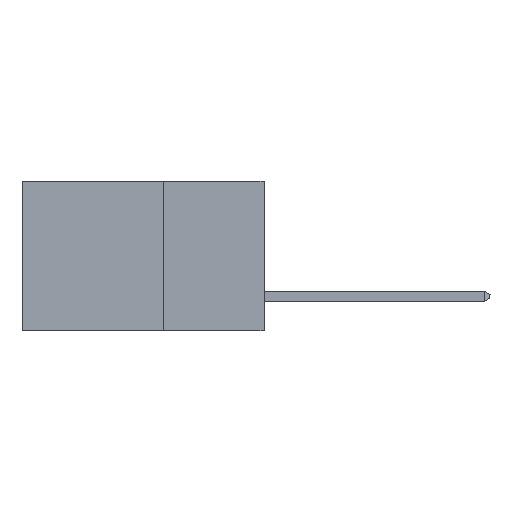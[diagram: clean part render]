
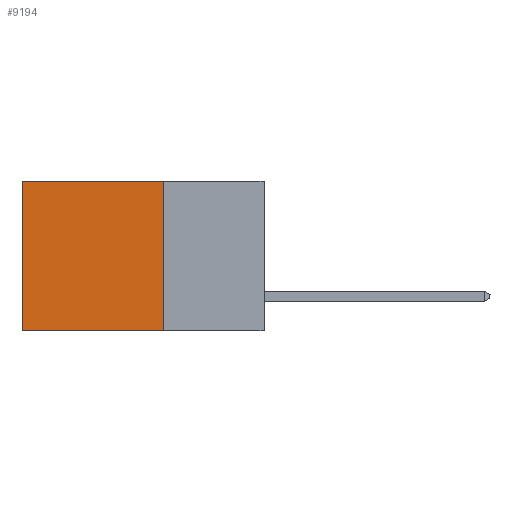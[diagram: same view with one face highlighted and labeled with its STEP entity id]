
A CAD part, left-side view. The second image highlights one B-rep face of the part: STEP entity #9194.
In plain terms, the highlighted planar face has unit normal (-1, 0, 0).
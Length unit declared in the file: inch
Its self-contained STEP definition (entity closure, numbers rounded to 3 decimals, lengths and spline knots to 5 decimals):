
#449 = EDGE_CURVE ( 'NONE', #10419, #15321, #13853, .T. ) ;
#1300 = ORIENTED_EDGE ( 'NONE', *, *, #17757, .F. ) ;
#1736 = LINE ( 'NONE', #4961, #5844 ) ;
#3112 = VECTOR ( 'NONE', #6103, 39.37008 ) ;
#3169 = CARTESIAN_POINT ( 'NONE',  ( 0.298, 0.6, 0. ) ) ;
#3438 = DIRECTION ( 'NONE',  ( 0., 1., 0. ) ) ;
#4318 = CARTESIAN_POINT ( 'NONE',  ( 0.298, 0.6, -0.37 ) ) ;
#4508 = VECTOR ( 'NONE', #12727, 39.37008 ) ;
#4566 = CARTESIAN_POINT ( 'NONE',  ( 0.298, 0.25, -0.37 ) ) ;
#4961 = CARTESIAN_POINT ( 'NONE',  ( 0.298, 0.25, 0. ) ) ;
#5080 = CARTESIAN_POINT ( 'NONE',  ( 0.298, 0.6, 0. ) ) ;
#5844 = VECTOR ( 'NONE', #3438, 39.37008 ) ;
#6103 = DIRECTION ( 'NONE',  ( 0., 0., -1. ) ) ;
#6957 = ORIENTED_EDGE ( 'NONE', *, *, #13905, .F. ) ;
#7982 = FACE_OUTER_BOUND ( 'NONE', #10154, .T. ) ;
#8925 = CARTESIAN_POINT ( 'NONE',  ( 0.298, 0.25, 0. ) ) ;
#9106 = LINE ( 'NONE', #9954, #4508 ) ;
#9194 = ADVANCED_FACE ( 'NONE', ( #7982 ), #15912, .F. ) ;
#9954 = CARTESIAN_POINT ( 'NONE',  ( 0.298, 0.25, -0.37 ) ) ;
#10154 = EDGE_LOOP ( 'NONE', ( #11232, #1300, #6957, #13799 ) ) ;
#10279 = EDGE_CURVE ( 'NONE', #11147, #10419, #1736, .T. ) ;
#10419 = VERTEX_POINT ( 'NONE', #5080 ) ;
#11147 = VERTEX_POINT ( 'NONE', #8925 ) ;
#11232 = ORIENTED_EDGE ( 'NONE', *, *, #449, .T. ) ;
#11244 = VERTEX_POINT ( 'NONE', #4566 ) ;
#11312 = DIRECTION ( 'NONE',  ( 0., 0., -1. ) ) ;
#12727 = DIRECTION ( 'NONE',  ( 0., 1., 0. ) ) ;
#12882 = DIRECTION ( 'NONE',  ( 1., 0., 0. ) ) ;
#13799 = ORIENTED_EDGE ( 'NONE', *, *, #10279, .T. ) ;
#13853 = LINE ( 'NONE', #3169, #3112 ) ;
#13905 = EDGE_CURVE ( 'NONE', #11147, #11244, #14624, .T. ) ;
#14624 = LINE ( 'NONE', #15257, #16191 ) ;
#14885 = AXIS2_PLACEMENT_3D ( 'NONE', #17222, #12882, #11312 ) ;
#15257 = CARTESIAN_POINT ( 'NONE',  ( 0.298, 0.25, 0. ) ) ;
#15321 = VERTEX_POINT ( 'NONE', #4318 ) ;
#15912 = PLANE ( 'NONE',  #14885 ) ;
#16191 = VECTOR ( 'NONE', #16471, 39.37008 ) ;
#16471 = DIRECTION ( 'NONE',  ( 0., 0., -1. ) ) ;
#17222 = CARTESIAN_POINT ( 'NONE',  ( 0.298, 0.25, 0. ) ) ;
#17757 = EDGE_CURVE ( 'NONE', #11244, #15321, #9106, .T. ) ;
